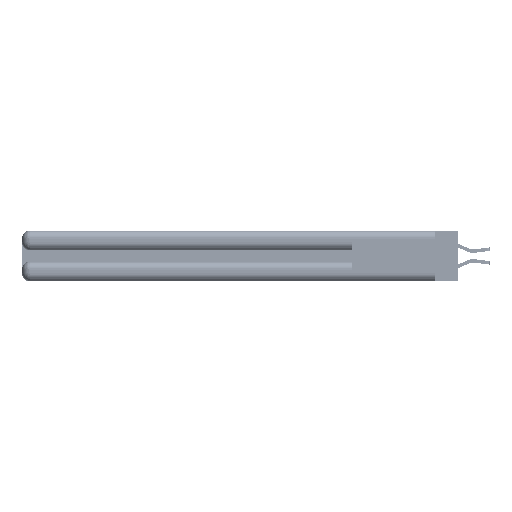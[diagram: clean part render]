
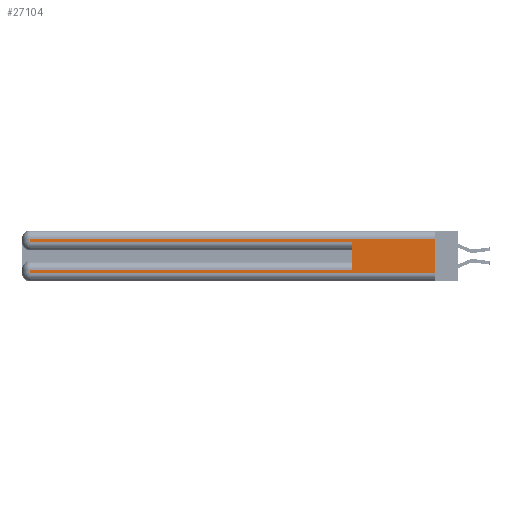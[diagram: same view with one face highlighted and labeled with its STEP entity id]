
A CAD part, left-side view. The second image highlights one B-rep face of the part: STEP entity #27104.
In plain terms, the highlighted planar face has unit normal (-1, 0, 0).
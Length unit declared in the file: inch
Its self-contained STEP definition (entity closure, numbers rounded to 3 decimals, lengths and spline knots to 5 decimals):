
#1083 = CARTESIAN_POINT ( 'NONE',  ( 0., 2.94, 0.37 ) ) ;
#2587 = VECTOR ( 'NONE', #45927, 39.37008 ) ;
#2697 = CARTESIAN_POINT ( 'NONE',  ( 0., 2.94, 0.06 ) ) ;
#3156 = VECTOR ( 'NONE', #10995, 39.37008 ) ;
#3227 = VERTEX_POINT ( 'NONE', #9693 ) ;
#3409 = CARTESIAN_POINT ( 'NONE',  ( 0., 0.6, 0.285 ) ) ;
#3722 = LINE ( 'NONE', #32895, #40134 ) ;
#4306 = LINE ( 'NONE', #7342, #3156 ) ;
#4877 = ORIENTED_EDGE ( 'NONE', *, *, #9333, .T. ) ;
#5395 = EDGE_CURVE ( 'NONE', #45923, #36071, #44337, .T. ) ;
#6924 = VERTEX_POINT ( 'NONE', #29158 ) ;
#7342 = CARTESIAN_POINT ( 'NONE',  ( 0., 0., 0.37 ) ) ;
#7345 = EDGE_LOOP ( 'NONE', ( #45053, #42214, #20101, #7604, #41751, #16240, #29781, #4877 ) ) ;
#7604 = ORIENTED_EDGE ( 'NONE', *, *, #5395, .T. ) ;
#8520 = LINE ( 'NONE', #1083, #43766 ) ;
#9333 = EDGE_CURVE ( 'NONE', #42248, #43028, #23084, .T. ) ;
#9693 = CARTESIAN_POINT ( 'NONE',  ( 0., 0.6, 0.085 ) ) ;
#10995 = DIRECTION ( 'NONE',  ( 0., 0., -1. ) ) ;
#11216 = LINE ( 'NONE', #43710, #19798 ) ;
#11218 = VERTEX_POINT ( 'NONE', #40756 ) ;
#12468 = CARTESIAN_POINT ( 'NONE',  ( 0., 0., 0.31 ) ) ;
#12489 = VERTEX_POINT ( 'NONE', #18576 ) ;
#13155 = DIRECTION ( 'NONE',  ( 0., -1., 0. ) ) ;
#16216 = LINE ( 'NONE', #12468, #24704 ) ;
#16240 = ORIENTED_EDGE ( 'NONE', *, *, #32161, .T. ) ;
#17408 = DIRECTION ( 'NONE',  ( 0., 0., -1. ) ) ;
#18576 = CARTESIAN_POINT ( 'NONE',  ( 0., 2.94, 0.31 ) ) ;
#19798 = VECTOR ( 'NONE', #25585, 39.37008 ) ;
#20048 = EDGE_CURVE ( 'NONE', #6924, #12489, #16216, .T. ) ;
#20101 = ORIENTED_EDGE ( 'NONE', *, *, #25756, .T. ) ;
#22421 = EDGE_CURVE ( 'NONE', #3227, #36071, #3722, .T. ) ;
#23084 = LINE ( 'NONE', #42272, #2587 ) ;
#23265 = DIRECTION ( 'NONE',  ( 0., 1., 0. ) ) ;
#24535 = PLANE ( 'NONE',  #28807 ) ;
#24704 = VECTOR ( 'NONE', #23265, 39.37008 ) ;
#25585 = DIRECTION ( 'NONE',  ( 0., 0., -1. ) ) ;
#25756 = EDGE_CURVE ( 'NONE', #12489, #45923, #8520, .T. ) ;
#27104 = ADVANCED_FACE ( 'NONE', ( #44777 ), #24535, .F. ) ;
#28807 = AXIS2_PLACEMENT_3D ( 'NONE', #31804, #39145, #17408 ) ;
#28947 = CARTESIAN_POINT ( 'NONE',  ( 0., 0., 0.085 ) ) ;
#29158 = CARTESIAN_POINT ( 'NONE',  ( 0., 0., 0.31 ) ) ;
#29781 = ORIENTED_EDGE ( 'NONE', *, *, #44350, .T. ) ;
#30143 = DIRECTION ( 'NONE',  ( 0., 0., -1. ) ) ;
#31496 = CARTESIAN_POINT ( 'NONE',  ( 0., 2.94, 0.285 ) ) ;
#31804 = CARTESIAN_POINT ( 'NONE',  ( 0., 0., 0.37 ) ) ;
#32161 = EDGE_CURVE ( 'NONE', #3227, #11218, #44856, .T. ) ;
#32811 = DIRECTION ( 'NONE',  ( 0., 1., 0. ) ) ;
#32895 = CARTESIAN_POINT ( 'NONE',  ( 0., 0.6, 0.145 ) ) ;
#34678 = VECTOR ( 'NONE', #13155, 39.37008 ) ;
#36071 = VERTEX_POINT ( 'NONE', #3409 ) ;
#36552 = DIRECTION ( 'NONE',  ( 0., 0., 1. ) ) ;
#36660 = CARTESIAN_POINT ( 'NONE',  ( 0., 0., 0.06 ) ) ;
#39145 = DIRECTION ( 'NONE',  ( 1., 0., 0. ) ) ;
#40134 = VECTOR ( 'NONE', #36552, 39.37008 ) ;
#40756 = CARTESIAN_POINT ( 'NONE',  ( 0., 2.94, 0.085 ) ) ;
#41445 = VECTOR ( 'NONE', #32811, 39.37008 ) ;
#41751 = ORIENTED_EDGE ( 'NONE', *, *, #22421, .F. ) ;
#42209 = CARTESIAN_POINT ( 'NONE',  ( 0., 0., 0.285 ) ) ;
#42214 = ORIENTED_EDGE ( 'NONE', *, *, #20048, .T. ) ;
#42248 = VERTEX_POINT ( 'NONE', #2697 ) ;
#42272 = CARTESIAN_POINT ( 'NONE',  ( 0., 0., 0.06 ) ) ;
#43028 = VERTEX_POINT ( 'NONE', #36660 ) ;
#43710 = CARTESIAN_POINT ( 'NONE',  ( 0., 2.94, 0.37 ) ) ;
#43766 = VECTOR ( 'NONE', #30143, 39.37008 ) ;
#44337 = LINE ( 'NONE', #42209, #34678 ) ;
#44350 = EDGE_CURVE ( 'NONE', #11218, #42248, #11216, .T. ) ;
#44777 = FACE_OUTER_BOUND ( 'NONE', #7345, .T. ) ;
#44856 = LINE ( 'NONE', #28947, #41445 ) ;
#45053 = ORIENTED_EDGE ( 'NONE', *, *, #46158, .F. ) ;
#45923 = VERTEX_POINT ( 'NONE', #31496 ) ;
#45927 = DIRECTION ( 'NONE',  ( 0., -1., 0. ) ) ;
#46158 = EDGE_CURVE ( 'NONE', #6924, #43028, #4306, .T. ) ;
